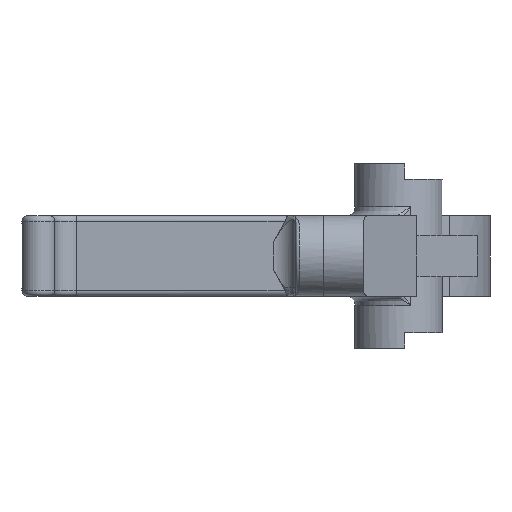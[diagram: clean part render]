
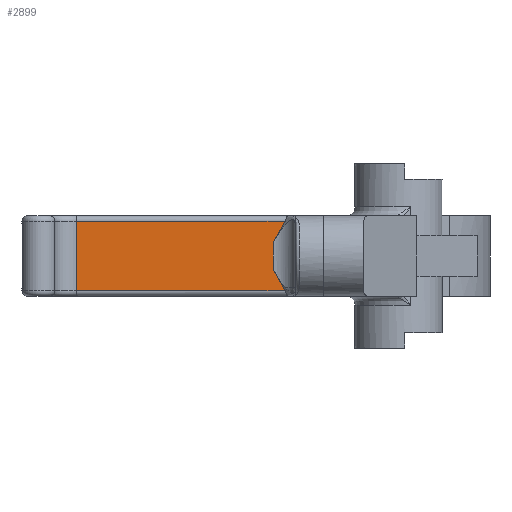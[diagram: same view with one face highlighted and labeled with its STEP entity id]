
A CAD part, left-side view. The second image highlights one B-rep face of the part: STEP entity #2899.
In plain terms, the highlighted planar face has unit normal (-1, 0, 0).
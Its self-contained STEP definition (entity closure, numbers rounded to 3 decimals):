
#145=FACE_OUTER_BOUND('',#311,.T.);
#311=EDGE_LOOP('',(#1991,#1992,#1993,#1994,#1995,#1996));
#473=LINE('',#4315,#691);
#486=LINE('',#9103,#704);
#487=LINE('',#9105,#705);
#488=LINE('',#9106,#706);
#691=VECTOR('',#3406,10.);
#704=VECTOR('',#3471,10.);
#705=VECTOR('',#3474,10.);
#706=VECTOR('',#3475,10.);
#911=B_SPLINE_CURVE_WITH_KNOTS('',3,(#6700,#6701,#6702,#6703,#6704,#6705,
#6706,#6707),.UNSPECIFIED.,.F.,.F.,(4,2,2,4),(0.057,0.101,
0.218,0.281),.UNSPECIFIED.);
#917=B_SPLINE_CURVE_WITH_KNOTS('',3,(#9061,#9062,#9063,#9064,#9065,#9066,
#9067,#9068),.UNSPECIFIED.,.F.,.F.,(4,2,2,4),(0.777,0.802,
0.872,0.931),.UNSPECIFIED.);
#1159=VERTEX_POINT('',#4290);
#1160=VERTEX_POINT('',#4314);
#1169=VERTEX_POINT('',#6676);
#1170=VERTEX_POINT('',#6699);
#1174=VERTEX_POINT('',#9052);
#1183=VERTEX_POINT('',#9096);
#1458=EDGE_CURVE('',#1159,#1160,#473,.T.);
#1473=EDGE_CURVE('',#1170,#1169,#911,.T.);
#1481=EDGE_CURVE('',#1159,#1174,#917,.T.);
#1498=EDGE_CURVE('',#1183,#1169,#486,.T.);
#1499=EDGE_CURVE('',#1160,#1183,#487,.T.);
#1500=EDGE_CURVE('',#1170,#1174,#488,.T.);
#1991=ORIENTED_EDGE('',*,*,#1498,.F.);
#1992=ORIENTED_EDGE('',*,*,#1499,.F.);
#1993=ORIENTED_EDGE('',*,*,#1458,.F.);
#1994=ORIENTED_EDGE('',*,*,#1481,.T.);
#1995=ORIENTED_EDGE('',*,*,#1500,.F.);
#1996=ORIENTED_EDGE('',*,*,#1473,.T.);
#2823=PLANE('',#3100);
#2899=ADVANCED_FACE('',(#145),#2823,.T.);
#3100=AXIS2_PLACEMENT_3D('',#9104,#3472,#3473);
#3406=DIRECTION('',(0.,1.,0.));
#3471=DIRECTION('',(0.,-1.,0.));
#3472=DIRECTION('center_axis',(-1.,0.,0.));
#3473=DIRECTION('ref_axis',(0.,-1.,0.));
#3474=DIRECTION('',(0.,0.,1.));
#3475=DIRECTION('',(0.,0.,-1.));
#4290=CARTESIAN_POINT('',(76.,3.537,-3.183));
#4314=CARTESIAN_POINT('',(76.,22.616,-3.183));
#4315=CARTESIAN_POINT('',(76.,8.07,-3.183));
#6676=CARTESIAN_POINT('',(76.,3.537,3.183));
#6699=CARTESIAN_POINT('',(76.,4.616,1.233));
#6700=CARTESIAN_POINT('Ctrl Pts',(76.,4.616,1.233));
#6701=CARTESIAN_POINT('Ctrl Pts',(76.,4.547,1.36));
#6702=CARTESIAN_POINT('Ctrl Pts',(76.,4.478,1.487));
#6703=CARTESIAN_POINT('Ctrl Pts',(76.,4.22,1.957));
#6704=CARTESIAN_POINT('Ctrl Pts',(76.,4.031,2.298));
#6705=CARTESIAN_POINT('Ctrl Pts',(76.,3.743,2.815));
#6706=CARTESIAN_POINT('Ctrl Pts',(76.,3.64,3.));
#6707=CARTESIAN_POINT('Ctrl Pts',(76.,3.537,3.183));
#9052=CARTESIAN_POINT('',(76.,4.616,-1.233));
#9061=CARTESIAN_POINT('Ctrl Pts',(76.,3.537,-3.183));
#9062=CARTESIAN_POINT('Ctrl Pts',(76.,3.595,-3.079));
#9063=CARTESIAN_POINT('Ctrl Pts',(76.,3.654,-2.975));
#9064=CARTESIAN_POINT('Ctrl Pts',(76.,3.875,-2.578));
#9065=CARTESIAN_POINT('Ctrl Pts',(76.,4.043,-2.277));
#9066=CARTESIAN_POINT('Ctrl Pts',(76.,4.345,-1.73));
#9067=CARTESIAN_POINT('Ctrl Pts',(76.,4.48,-1.484));
#9068=CARTESIAN_POINT('Ctrl Pts',(76.,4.616,-1.233));
#9096=CARTESIAN_POINT('',(76.,22.616,3.183));
#9103=CARTESIAN_POINT('',(76.,19.848,3.183));
#9104=CARTESIAN_POINT('Origin',(76.,24.616,-3.683));
#9105=CARTESIAN_POINT('',(76.,22.616,-3.683));
#9106=CARTESIAN_POINT('',(76.,4.616,-8.192));
